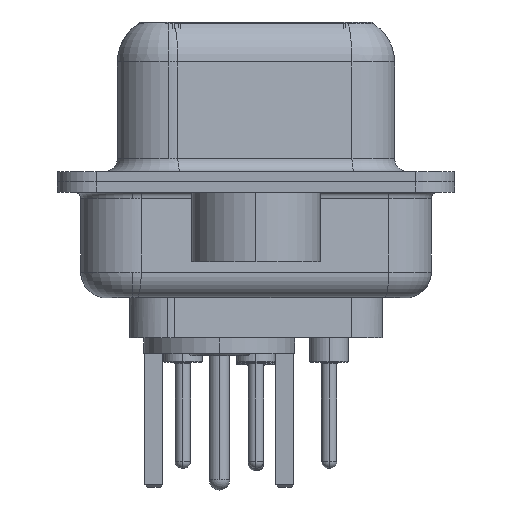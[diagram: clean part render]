
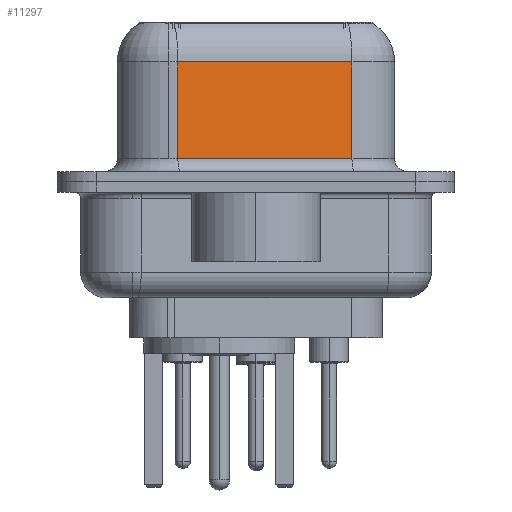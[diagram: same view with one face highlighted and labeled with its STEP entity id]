
A CAD part, left-side view. The second image highlights one B-rep face of the part: STEP entity #11297.
In plain terms, the highlighted planar face has unit normal (-0.985, -0.174, 0).
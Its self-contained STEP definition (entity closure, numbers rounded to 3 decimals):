
#167 = DIRECTION ( 'NONE',  ( 0., 0., -1. ) ) ;
#586 = AXIS2_PLACEMENT_3D ( 'NONE', #26139, #32459, #2371 ) ;
#2371 = DIRECTION ( 'NONE',  ( -0.174, 0.985, 0. ) ) ;
#2972 = VERTEX_POINT ( 'NONE', #9583 ) ;
#2988 = ORIENTED_EDGE ( 'NONE', *, *, #18355, .F. ) ;
#4142 = LINE ( 'NONE', #5199, #20769 ) ;
#5199 = CARTESIAN_POINT ( 'NONE',  ( 4.43, 3.028, 6.4 ) ) ;
#6142 = DIRECTION ( 'NONE',  ( -0.174, 0.985, 0. ) ) ;
#6383 = CARTESIAN_POINT ( 'NONE',  ( 5.621, -3.722, 4.65 ) ) ;
#6628 = EDGE_CURVE ( 'NONE', #19119, #30283, #21591, .T. ) ;
#7406 = EDGE_CURVE ( 'NONE', #2972, #16630, #21111, .T. ) ;
#9583 = CARTESIAN_POINT ( 'NONE',  ( 5.621, -3.722, 4.65 ) ) ;
#11297 = ADVANCED_FACE ( 'NONE', ( #14541 ), #17775, .F. ) ;
#14541 = FACE_OUTER_BOUND ( 'NONE', #25558, .T. ) ;
#14882 = CARTESIAN_POINT ( 'NONE',  ( 4.43, 3.028, 0.9 ) ) ;
#15147 = VECTOR ( 'NONE', #6142, 1000. ) ;
#15977 = DIRECTION ( 'NONE',  ( 0., 0., -1. ) ) ;
#16630 = VERTEX_POINT ( 'NONE', #28021 ) ;
#17775 = PLANE ( 'NONE',  #586 ) ;
#17904 = ORIENTED_EDGE ( 'NONE', *, *, #6628, .T. ) ;
#18355 = EDGE_CURVE ( 'NONE', #2972, #30283, #24329, .T. ) ;
#19119 = VERTEX_POINT ( 'NONE', #14882 ) ;
#20769 = VECTOR ( 'NONE', #15977, 1000. ) ;
#21111 = LINE ( 'NONE', #6383, #15147 ) ;
#21519 = CARTESIAN_POINT ( 'NONE',  ( 5.621, -3.722, 0.9 ) ) ;
#21591 = LINE ( 'NONE', #21519, #34005 ) ;
#22255 = CARTESIAN_POINT ( 'NONE',  ( 5.621, -3.722, 6.4 ) ) ;
#24284 = DIRECTION ( 'NONE',  ( 0.174, -0.985, 0. ) ) ;
#24329 = LINE ( 'NONE', #22255, #25648 ) ;
#25558 = EDGE_LOOP ( 'NONE', ( #2988, #32239, #25692, #17904 ) ) ;
#25648 = VECTOR ( 'NONE', #167, 1000. ) ;
#25692 = ORIENTED_EDGE ( 'NONE', *, *, #33745, .T. ) ;
#26139 = CARTESIAN_POINT ( 'NONE',  ( 5.621, -3.722, 6.4 ) ) ;
#27271 = CARTESIAN_POINT ( 'NONE',  ( 5.621, -3.722, 0.9 ) ) ;
#28021 = CARTESIAN_POINT ( 'NONE',  ( 4.43, 3.028, 4.65 ) ) ;
#30283 = VERTEX_POINT ( 'NONE', #27271 ) ;
#32239 = ORIENTED_EDGE ( 'NONE', *, *, #7406, .T. ) ;
#32459 = DIRECTION ( 'NONE',  ( 0.985, 0.174, 0. ) ) ;
#33745 = EDGE_CURVE ( 'NONE', #16630, #19119, #4142, .T. ) ;
#34005 = VECTOR ( 'NONE', #24284, 1000. ) ;
